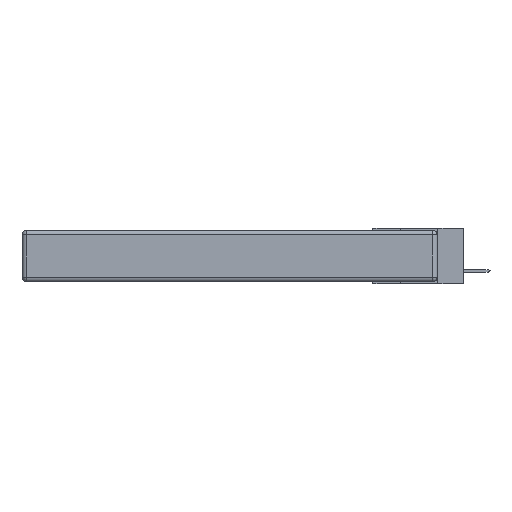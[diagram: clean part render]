
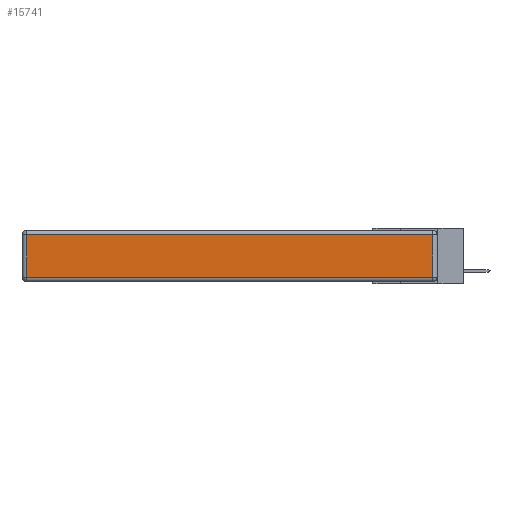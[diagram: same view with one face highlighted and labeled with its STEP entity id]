
A CAD part, left-side view. The second image highlights one B-rep face of the part: STEP entity #15741.
In plain terms, the highlighted planar face has unit normal (-1, 0, 0).
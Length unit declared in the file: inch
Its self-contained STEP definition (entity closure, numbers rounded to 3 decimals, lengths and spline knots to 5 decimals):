
#340 = ORIENTED_EDGE ( 'NONE', *, *, #18306, .T. ) ;
#982 = PLANE ( 'NONE',  #11855 ) ;
#1295 = CARTESIAN_POINT ( 'NONE',  ( 0., 0., -0.343 ) ) ;
#2673 = VECTOR ( 'NONE', #4725, 39.37008 ) ;
#3486 = CARTESIAN_POINT ( 'NONE',  ( 0., 2.72, -0.313 ) ) ;
#4402 = CARTESIAN_POINT ( 'NONE',  ( 0., 0., -0.313 ) ) ;
#4725 = DIRECTION ( 'NONE',  ( 0., 0., -1. ) ) ;
#5504 = DIRECTION ( 'NONE',  ( 0., 0., 1. ) ) ;
#5899 = LINE ( 'NONE', #4402, #17079 ) ;
#6872 = VERTEX_POINT ( 'NONE', #16349 ) ;
#7782 = DIRECTION ( 'NONE',  ( 0., 0., 1. ) ) ;
#8274 = EDGE_LOOP ( 'NONE', ( #9499, #340, #14917, #10435 ) ) ;
#8301 = DIRECTION ( 'NONE',  ( 0., 1., 0. ) ) ;
#8453 = VERTEX_POINT ( 'NONE', #3486 ) ;
#8841 = LINE ( 'NONE', #10572, #12221 ) ;
#9499 = ORIENTED_EDGE ( 'NONE', *, *, #12756, .T. ) ;
#10435 = ORIENTED_EDGE ( 'NONE', *, *, #14413, .T. ) ;
#10572 = CARTESIAN_POINT ( 'NONE',  ( 0., 0.03, -0.343 ) ) ;
#11291 = CARTESIAN_POINT ( 'NONE',  ( 0., 0.03, -0.03 ) ) ;
#11379 = DIRECTION ( 'NONE',  ( -1., 0., 0. ) ) ;
#11802 = VECTOR ( 'NONE', #8301, 39.37008 ) ;
#11845 = DIRECTION ( 'NONE',  ( 0., -1., 0. ) ) ;
#11855 = AXIS2_PLACEMENT_3D ( 'NONE', #1295, #11379, #5504 ) ;
#11988 = CARTESIAN_POINT ( 'NONE',  ( 0., 2.72, -0.343 ) ) ;
#12221 = VECTOR ( 'NONE', #7782, 39.37008 ) ;
#12715 = LINE ( 'NONE', #17064, #11802 ) ;
#12756 = EDGE_CURVE ( 'NONE', #8453, #6872, #5899, .T. ) ;
#13572 = LINE ( 'NONE', #11988, #2673 ) ;
#14238 = FACE_OUTER_BOUND ( 'NONE', #8274, .T. ) ;
#14413 = EDGE_CURVE ( 'NONE', #18774, #8453, #13572, .T. ) ;
#14917 = ORIENTED_EDGE ( 'NONE', *, *, #17627, .T. ) ;
#15741 = ADVANCED_FACE ( 'NONE', ( #14238 ), #982, .T. ) ;
#16349 = CARTESIAN_POINT ( 'NONE',  ( 0., 0.03, -0.313 ) ) ;
#16594 = VERTEX_POINT ( 'NONE', #11291 ) ;
#16859 = CARTESIAN_POINT ( 'NONE',  ( 0., 2.72, -0.03 ) ) ;
#17064 = CARTESIAN_POINT ( 'NONE',  ( 0., 2.75, -0.03 ) ) ;
#17079 = VECTOR ( 'NONE', #11845, 39.37008 ) ;
#17627 = EDGE_CURVE ( 'NONE', #16594, #18774, #12715, .T. ) ;
#18306 = EDGE_CURVE ( 'NONE', #6872, #16594, #8841, .T. ) ;
#18774 = VERTEX_POINT ( 'NONE', #16859 ) ;
